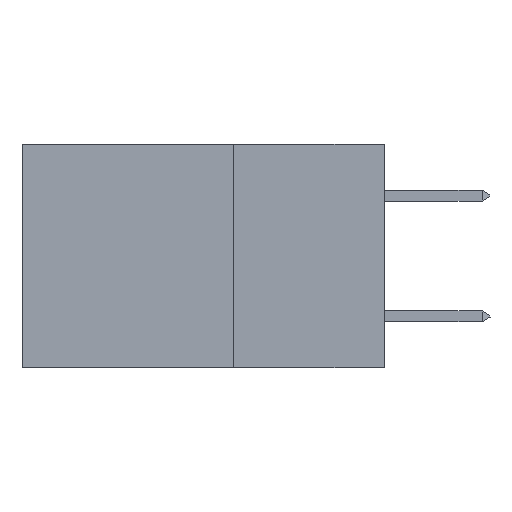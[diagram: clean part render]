
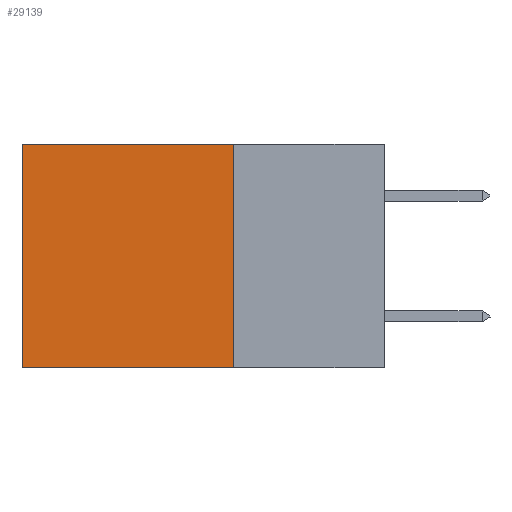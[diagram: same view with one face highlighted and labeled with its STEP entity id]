
A CAD part, left-side view. The second image highlights one B-rep face of the part: STEP entity #29139.
In plain terms, the highlighted planar face has unit normal (-1, 0, 0).
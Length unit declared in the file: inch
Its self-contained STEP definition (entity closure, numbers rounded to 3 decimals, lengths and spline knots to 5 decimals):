
#1289 = DIRECTION ( 'NONE',  ( 0., 0., -1. ) ) ;
#1492 = VECTOR ( 'NONE', #3050, 39.37008 ) ;
#1991 = LINE ( 'NONE', #29226, #27882 ) ;
#2228 = ORIENTED_EDGE ( 'NONE', *, *, #19331, .T. ) ;
#3050 = DIRECTION ( 'NONE',  ( 0., 1., 0. ) ) ;
#3076 = AXIS2_PLACEMENT_3D ( 'NONE', #20227, #12813, #5406 ) ;
#5406 = DIRECTION ( 'NONE',  ( 0., 0., -1. ) ) ;
#6585 = CARTESIAN_POINT ( 'NONE',  ( 0.2875, 0.25, -0.37 ) ) ;
#6941 = EDGE_CURVE ( 'NONE', #26287, #12368, #16766, .T. ) ;
#7211 = FACE_OUTER_BOUND ( 'NONE', #32178, .T. ) ;
#7297 = DIRECTION ( 'NONE',  ( 0., 0., -1. ) ) ;
#10107 = CARTESIAN_POINT ( 'NONE',  ( 0.2875, 0.6, 0. ) ) ;
#11472 = ORIENTED_EDGE ( 'NONE', *, *, #6941, .F. ) ;
#11540 = LINE ( 'NONE', #24719, #21028 ) ;
#11788 = EDGE_CURVE ( 'NONE', #31229, #26287, #1991, .T. ) ;
#12368 = VERTEX_POINT ( 'NONE', #17445 ) ;
#12813 = DIRECTION ( 'NONE',  ( 1., 0., 0. ) ) ;
#16766 = LINE ( 'NONE', #28278, #1492 ) ;
#17445 = CARTESIAN_POINT ( 'NONE',  ( 0.2875, 0.6, -0.37 ) ) ;
#18552 = EDGE_CURVE ( 'NONE', #31229, #29890, #11540, .T. ) ;
#19331 = EDGE_CURVE ( 'NONE', #29890, #12368, #25057, .T. ) ;
#20227 = CARTESIAN_POINT ( 'NONE',  ( 0.2875, 0.25, 0. ) ) ;
#21028 = VECTOR ( 'NONE', #22294, 39.37008 ) ;
#22294 = DIRECTION ( 'NONE',  ( 0., 1., 0. ) ) ;
#22596 = CARTESIAN_POINT ( 'NONE',  ( 0.2875, 0.25, 0. ) ) ;
#22874 = PLANE ( 'NONE',  #3076 ) ;
#24719 = CARTESIAN_POINT ( 'NONE',  ( 0.2875, 0.25, 0. ) ) ;
#25057 = LINE ( 'NONE', #10107, #30890 ) ;
#26287 = VERTEX_POINT ( 'NONE', #6585 ) ;
#27271 = ORIENTED_EDGE ( 'NONE', *, *, #18552, .T. ) ;
#27882 = VECTOR ( 'NONE', #1289, 39.37008 ) ;
#28278 = CARTESIAN_POINT ( 'NONE',  ( 0.2875, 0.25, -0.37 ) ) ;
#29139 = ADVANCED_FACE ( 'NONE', ( #7211 ), #22874, .F. ) ;
#29226 = CARTESIAN_POINT ( 'NONE',  ( 0.2875, 0.25, 0. ) ) ;
#29349 = CARTESIAN_POINT ( 'NONE',  ( 0.2875, 0.6, 0. ) ) ;
#29890 = VERTEX_POINT ( 'NONE', #29349 ) ;
#30890 = VECTOR ( 'NONE', #7297, 39.37008 ) ;
#31229 = VERTEX_POINT ( 'NONE', #22596 ) ;
#31531 = ORIENTED_EDGE ( 'NONE', *, *, #11788, .F. ) ;
#32178 = EDGE_LOOP ( 'NONE', ( #2228, #11472, #31531, #27271 ) ) ;
